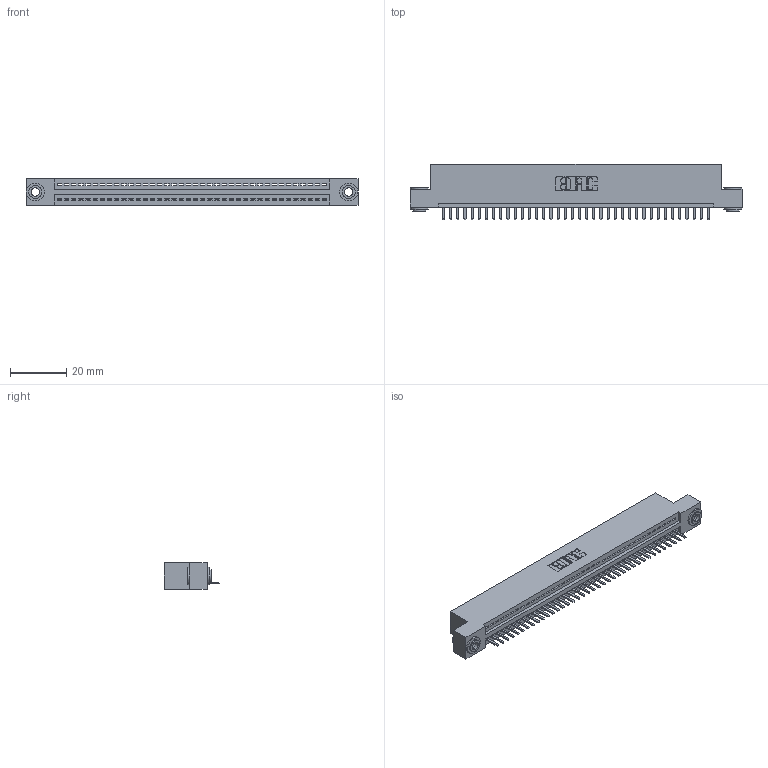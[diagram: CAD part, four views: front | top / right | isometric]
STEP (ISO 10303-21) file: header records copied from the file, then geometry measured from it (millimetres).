
FILE_DESCRIPTION (( 'STEP AP203' ), '1' );
FILE_NAME ('395-038-520-103.STEP', '2018-11-14T01:06:22', ( '' ), ( '' ), 'SwSTEP 2.0', 'SolidWorks 2016', '' );
FILE_SCHEMA (( 'CONFIG_CONTROL_DESIGN' ));
Length unit declared in the file: inch
Products named in the file (4): 395-038-520-103; 345-292-001_345-293-120; 345 Part_Flush Mounting Lugs - 0.156 Dia-TH; 345-250-002_345-250-002-102
Assembly tree (41 placements, depth 2):
  395-038-520-103
    345 Part_Flush Mounting Lugs - 0.156 Dia-TH
    345-292-001_345-293-120  x38
    345-250-002_345-250-002-102  x2
Bounding box: 117.73 x 19.68 x 9.4 mm (x, y, z)
Volume: 11059.3 mm3; surface area: 14499.4 mm2
Topology: 41 solids, 41 shells, 2520 faces, 7409 edges, 4834 vertices
Faces by surface type: plane 1686, cylinder 826, cone 8
Entity records: 29902 total; most frequent: CARTESIAN_POINT 5169, ORIENTED_EDGE 5122, DIRECTION 4539, EDGE_CURVE 2561, VECTOR 2249, LINE 2249, VERTEX_POINT 1702, AXIS2_PLACEMENT_3D 1145
